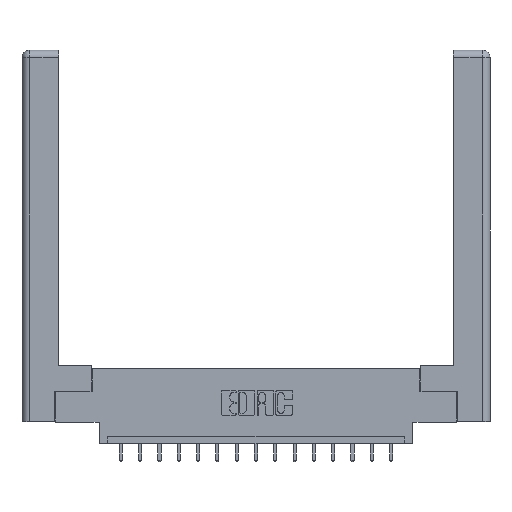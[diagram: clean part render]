
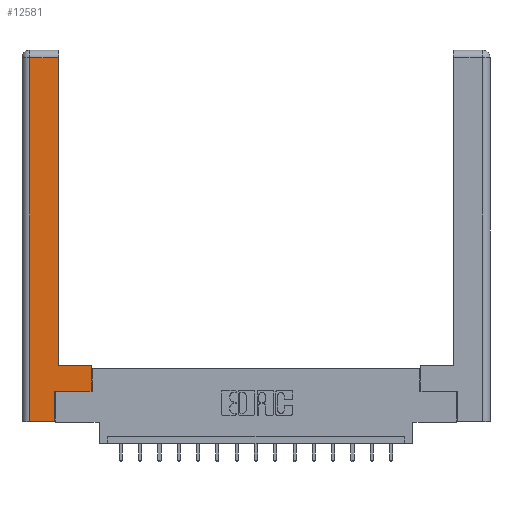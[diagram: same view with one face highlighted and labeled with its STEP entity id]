
A CAD part, top view. The second image highlights one B-rep face of the part: STEP entity #12581.
In plain terms, the highlighted planar face has unit normal (0, 0, 1).
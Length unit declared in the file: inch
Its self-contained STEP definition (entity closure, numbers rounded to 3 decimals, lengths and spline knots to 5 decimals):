
#66 = ORIENTED_EDGE ( 'NONE', *, *, #8544, .T. ) ;
#675 = CARTESIAN_POINT ( 'NONE',  ( 0.295, 0.45, 0. ) ) ;
#694 = ORIENTED_EDGE ( 'NONE', *, *, #15582, .T. ) ;
#1003 = VERTEX_POINT ( 'NONE', #3602 ) ;
#1368 = VECTOR ( 'NONE', #7062, 39.37008 ) ;
#1498 = EDGE_LOOP ( 'NONE', ( #11189, #694, #17334, #3793, #14376, #5157, #66, #4227 ) ) ;
#1747 = EDGE_CURVE ( 'NONE', #11406, #1003, #3869, .T. ) ;
#1927 = LINE ( 'NONE', #2508, #16254 ) ;
#2262 = EDGE_CURVE ( 'NONE', #3817, #11406, #3016, .T. ) ;
#2361 = LINE ( 'NONE', #11934, #8701 ) ;
#2415 = VECTOR ( 'NONE', #11426, 39.37008 ) ;
#2508 = CARTESIAN_POINT ( 'NONE',  ( 0.295, 3., 0. ) ) ;
#2743 = CARTESIAN_POINT ( 'NONE',  ( 0.295, 2.94, 0. ) ) ;
#3016 = LINE ( 'NONE', #16604, #1368 ) ;
#3302 = CARTESIAN_POINT ( 'NONE',  ( 0.0615, 2.94, 0. ) ) ;
#3471 = CARTESIAN_POINT ( 'NONE',  ( 0.0615, 0., 0. ) ) ;
#3602 = CARTESIAN_POINT ( 'NONE',  ( 0.565, 0.245, 0. ) ) ;
#3793 = ORIENTED_EDGE ( 'NONE', *, *, #5957, .T. ) ;
#3817 = VERTEX_POINT ( 'NONE', #15699 ) ;
#3869 = LINE ( 'NONE', #6071, #2415 ) ;
#3968 = VERTEX_POINT ( 'NONE', #675 ) ;
#4227 = ORIENTED_EDGE ( 'NONE', *, *, #17288, .T. ) ;
#4388 = VECTOR ( 'NONE', #14907, 39.37008 ) ;
#5157 = ORIENTED_EDGE ( 'NONE', *, *, #1747, .T. ) ;
#5249 = CARTESIAN_POINT ( 'NONE',  ( 0.565, 0.45, 0. ) ) ;
#5957 = EDGE_CURVE ( 'NONE', #13058, #3817, #6511, .T. ) ;
#6071 = CARTESIAN_POINT ( 'NONE',  ( 0.565, 0.245, 0. ) ) ;
#6511 = LINE ( 'NONE', #16047, #4388 ) ;
#6719 = DIRECTION ( 'NONE',  ( 0., 1., 0. ) ) ;
#6808 = PLANE ( 'NONE',  #13587 ) ;
#7062 = DIRECTION ( 'NONE',  ( 0., 1., 0. ) ) ;
#7434 = VECTOR ( 'NONE', #14624, 39.37008 ) ;
#7848 = CARTESIAN_POINT ( 'NONE',  ( 0., 0., 0. ) ) ;
#7898 = DIRECTION ( 'NONE',  ( 0., 0., -1. ) ) ;
#8544 = EDGE_CURVE ( 'NONE', #1003, #12562, #2361, .T. ) ;
#8701 = VECTOR ( 'NONE', #10659, 39.37008 ) ;
#9414 = FACE_OUTER_BOUND ( 'NONE', #1498, .T. ) ;
#10372 = CARTESIAN_POINT ( 'NONE',  ( 0.265, 0.245, 0. ) ) ;
#10659 = DIRECTION ( 'NONE',  ( 0., 1., 0. ) ) ;
#11189 = ORIENTED_EDGE ( 'NONE', *, *, #13998, .T. ) ;
#11406 = VERTEX_POINT ( 'NONE', #10372 ) ;
#11426 = DIRECTION ( 'NONE',  ( 1., 0., 0. ) ) ;
#11453 = VERTEX_POINT ( 'NONE', #2743 ) ;
#11649 = LINE ( 'NONE', #13264, #7434 ) ;
#11860 = DIRECTION ( 'NONE',  ( -1., 0., 0. ) ) ;
#11934 = CARTESIAN_POINT ( 'NONE',  ( 0.565, 0.45, 0. ) ) ;
#12562 = VERTEX_POINT ( 'NONE', #5249 ) ;
#12581 = ADVANCED_FACE ( 'NONE', ( #9414 ), #6808, .F. ) ;
#12690 = DIRECTION ( 'NONE',  ( -1., 0., 0. ) ) ;
#13058 = VERTEX_POINT ( 'NONE', #3471 ) ;
#13264 = CARTESIAN_POINT ( 'NONE',  ( 0.0615, 0., 0. ) ) ;
#13587 = AXIS2_PLACEMENT_3D ( 'NONE', #7848, #7898, #17358 ) ;
#13829 = EDGE_CURVE ( 'NONE', #16896, #13058, #11649, .T. ) ;
#13863 = VECTOR ( 'NONE', #12690, 39.37008 ) ;
#13998 = EDGE_CURVE ( 'NONE', #3968, #11453, #1927, .T. ) ;
#14376 = ORIENTED_EDGE ( 'NONE', *, *, #2262, .T. ) ;
#14553 = VECTOR ( 'NONE', #11860, 39.37008 ) ;
#14624 = DIRECTION ( 'NONE',  ( 0., -1., 0. ) ) ;
#14907 = DIRECTION ( 'NONE',  ( 1., 0., 0. ) ) ;
#15398 = LINE ( 'NONE', #16942, #14553 ) ;
#15582 = EDGE_CURVE ( 'NONE', #11453, #16896, #16608, .T. ) ;
#15699 = CARTESIAN_POINT ( 'NONE',  ( 0.265, 0., 0. ) ) ;
#16047 = CARTESIAN_POINT ( 'NONE',  ( 0.265, 0., 0. ) ) ;
#16254 = VECTOR ( 'NONE', #6719, 39.37008 ) ;
#16604 = CARTESIAN_POINT ( 'NONE',  ( 0.265, 0.245, 0. ) ) ;
#16608 = LINE ( 'NONE', #3302, #13863 ) ;
#16896 = VERTEX_POINT ( 'NONE', #16909 ) ;
#16909 = CARTESIAN_POINT ( 'NONE',  ( 0.0615, 2.94, 0. ) ) ;
#16942 = CARTESIAN_POINT ( 'NONE',  ( 0.295, 0.45, 0. ) ) ;
#17288 = EDGE_CURVE ( 'NONE', #12562, #3968, #15398, .T. ) ;
#17334 = ORIENTED_EDGE ( 'NONE', *, *, #13829, .T. ) ;
#17358 = DIRECTION ( 'NONE',  ( -1., 0., 0. ) ) ;
